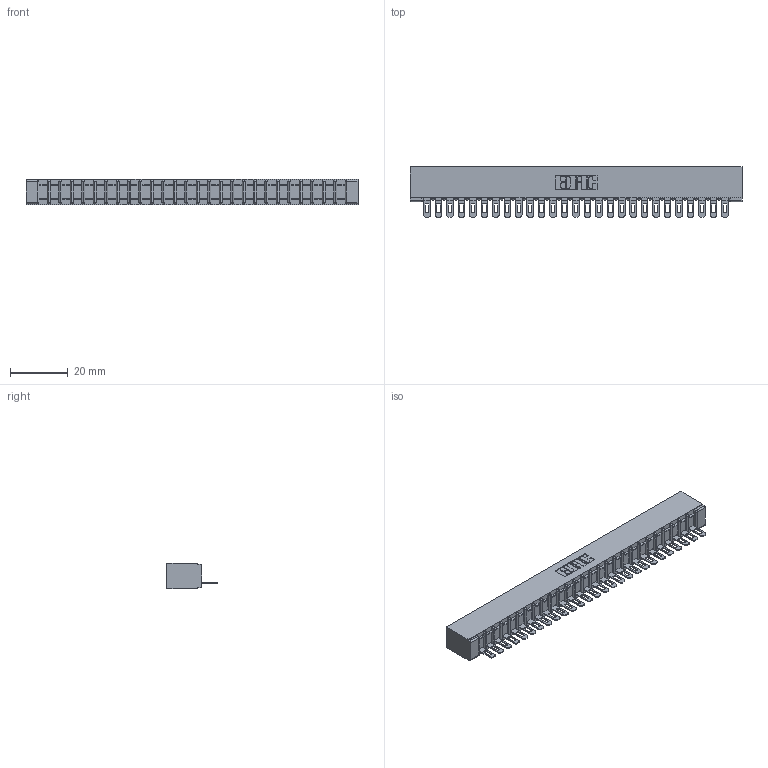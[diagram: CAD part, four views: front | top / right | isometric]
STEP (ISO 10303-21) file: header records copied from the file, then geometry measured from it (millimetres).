
FILE_DESCRIPTION (( 'STEP AP203' ), '1' );
FILE_NAME ('307-027-401-101.STEP', '2020-09-28T05:10:51', ( '' ), ( '' ), 'SwSTEP 2.0', 'SolidWorks 2020', '' );
FILE_SCHEMA (( 'CONFIG_CONTROL_DESIGN' ));
Length unit declared in the file: inch
Products named in the file (3): 307-027-401-101; 307 Part_No Mounting Lugs; 307-290-002_501
Assembly tree (28 placements, depth 2):
  307-027-401-101
    307 Part_No Mounting Lugs
    307-290-002_501  x27
Bounding box: 114.86 x 17.42 x 8.71 mm (x, y, z)
Volume: 7851.2 mm3; surface area: 15247 mm2
Topology: 28 solids, 28 shells, 2190 faces, 6725 edges, 4406 vertices
Faces by surface type: plane 1254, cylinder 880, sphere 56
Entity records: 25512 total; most frequent: CARTESIAN_POINT 4300, ORIENTED_EDGE 4290, DIRECTION 4187, EDGE_CURVE 2145, LINE 1633, VECTOR 1633, VERTEX_POINT 1390, AXIS2_PLACEMENT_3D 1277
